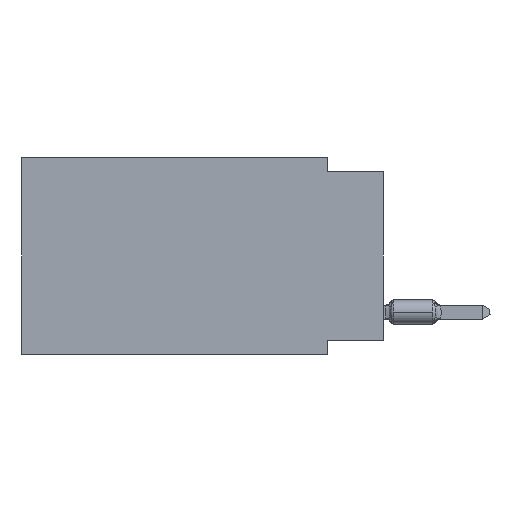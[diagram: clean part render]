
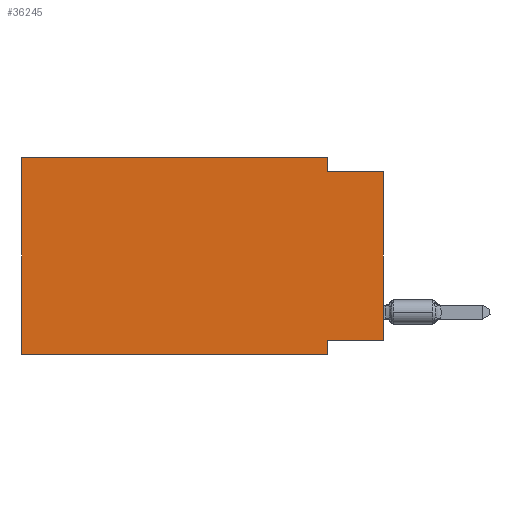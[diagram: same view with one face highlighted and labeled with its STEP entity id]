
A CAD part, left-side view. The second image highlights one B-rep face of the part: STEP entity #36245.
In plain terms, the highlighted planar face has unit normal (-1, 0, 0).
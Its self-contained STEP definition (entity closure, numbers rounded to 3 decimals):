
#801 = EDGE_CURVE ( 'NONE', #10428, #63160, #31707, .T. ) ;
#3510 = VECTOR ( 'NONE', #16672, 1000. ) ;
#4188 = CARTESIAN_POINT ( 'NONE',  ( 0., 0., -8.255 ) ) ;
#4580 = CARTESIAN_POINT ( 'NONE',  ( 0., 16.383, 0. ) ) ;
#5194 = FACE_OUTER_BOUND ( 'NONE', #32327, .T. ) ;
#7458 = CARTESIAN_POINT ( 'NONE',  ( 0., 0., -8.255 ) ) ;
#8635 = CARTESIAN_POINT ( 'NONE',  ( 0., 0., -0.635 ) ) ;
#9590 = CARTESIAN_POINT ( 'NONE',  ( 0., 16.383, 0. ) ) ;
#10428 = VERTEX_POINT ( 'NONE', #29338 ) ;
#11068 = CARTESIAN_POINT ( 'NONE',  ( 0., 2.54, -0.635 ) ) ;
#11115 = AXIS2_PLACEMENT_3D ( 'NONE', #39420, #14782, #29189 ) ;
#11839 = VERTEX_POINT ( 'NONE', #8635 ) ;
#14782 = DIRECTION ( 'NONE',  ( 1., 0., 0. ) ) ;
#16672 = DIRECTION ( 'NONE',  ( 0., 0., 1. ) ) ;
#18533 = LINE ( 'NONE', #28449, #47121 ) ;
#18869 = LINE ( 'NONE', #9590, #39000 ) ;
#18970 = ORIENTED_EDGE ( 'NONE', *, *, #21011, .F. ) ;
#19207 = CARTESIAN_POINT ( 'NONE',  ( 0., 2.54, 0. ) ) ;
#19904 = PLANE ( 'NONE',  #11115 ) ;
#20805 = DIRECTION ( 'NONE',  ( 0., 0., -1. ) ) ;
#21011 = EDGE_CURVE ( 'NONE', #24357, #11839, #50283, .T. ) ;
#21856 = EDGE_CURVE ( 'NONE', #10428, #28806, #18533, .T. ) ;
#22291 = VECTOR ( 'NONE', #33310, 1000. ) ;
#23144 = CARTESIAN_POINT ( 'NONE',  ( 0., 2.54, -8.89 ) ) ;
#23416 = ORIENTED_EDGE ( 'NONE', *, *, #34055, .F. ) ;
#24179 = CARTESIAN_POINT ( 'NONE',  ( 0., 2.54, -8.255 ) ) ;
#24357 = VERTEX_POINT ( 'NONE', #11068 ) ;
#26567 = DIRECTION ( 'NONE',  ( 0., -1., 0. ) ) ;
#28449 = CARTESIAN_POINT ( 'NONE',  ( 0., 16.383, -8.89 ) ) ;
#28806 = VERTEX_POINT ( 'NONE', #23144 ) ;
#29101 = DIRECTION ( 'NONE',  ( 0., -1., 0. ) ) ;
#29189 = DIRECTION ( 'NONE',  ( 0., 0., -1. ) ) ;
#29338 = CARTESIAN_POINT ( 'NONE',  ( 0., 16.383, -8.89 ) ) ;
#31707 = LINE ( 'NONE', #50925, #3510 ) ;
#32327 = EDGE_LOOP ( 'NONE', ( #61932, #18970, #61066, #52282, #50179, #55078, #33353, #23416 ) ) ;
#33310 = DIRECTION ( 'NONE',  ( 0., 1., 0. ) ) ;
#33353 = ORIENTED_EDGE ( 'NONE', *, *, #44861, .F. ) ;
#33989 = LINE ( 'NONE', #49350, #41806 ) ;
#34055 = EDGE_CURVE ( 'NONE', #34829, #39649, #52845, .T. ) ;
#34829 = VERTEX_POINT ( 'NONE', #7458 ) ;
#34842 = CARTESIAN_POINT ( 'NONE',  ( 0., 2.54, -8.89 ) ) ;
#34889 = CARTESIAN_POINT ( 'NONE',  ( 0., 2.54, 0. ) ) ;
#36245 = ADVANCED_FACE ( 'NONE', ( #5194 ), #19904, .F. ) ;
#36271 = EDGE_CURVE ( 'NONE', #34829, #11839, #33989, .T. ) ;
#36630 = VERTEX_POINT ( 'NONE', #19207 ) ;
#37724 = VECTOR ( 'NONE', #26567, 1000. ) ;
#39000 = VECTOR ( 'NONE', #29101, 1000. ) ;
#39420 = CARTESIAN_POINT ( 'NONE',  ( 0., 16.383, 0. ) ) ;
#39649 = VERTEX_POINT ( 'NONE', #24179 ) ;
#40978 = LINE ( 'NONE', #34889, #50881 ) ;
#41806 = VECTOR ( 'NONE', #49029, 1000. ) ;
#44258 = EDGE_CURVE ( 'NONE', #63160, #36630, #18869, .T. ) ;
#44861 = EDGE_CURVE ( 'NONE', #39649, #28806, #59173, .T. ) ;
#45470 = CARTESIAN_POINT ( 'NONE',  ( 0., 0., -0.635 ) ) ;
#47121 = VECTOR ( 'NONE', #48605, 1000. ) ;
#48605 = DIRECTION ( 'NONE',  ( 0., -1., 0. ) ) ;
#49029 = DIRECTION ( 'NONE',  ( 0., 0., 1. ) ) ;
#49350 = CARTESIAN_POINT ( 'NONE',  ( 0., 0., 0. ) ) ;
#50179 = ORIENTED_EDGE ( 'NONE', *, *, #801, .F. ) ;
#50283 = LINE ( 'NONE', #45470, #37724 ) ;
#50335 = VECTOR ( 'NONE', #54371, 1000. ) ;
#50881 = VECTOR ( 'NONE', #20805, 1000. ) ;
#50925 = CARTESIAN_POINT ( 'NONE',  ( 0., 16.383, 0. ) ) ;
#52282 = ORIENTED_EDGE ( 'NONE', *, *, #44258, .F. ) ;
#52845 = LINE ( 'NONE', #4188, #22291 ) ;
#54371 = DIRECTION ( 'NONE',  ( 0., 0., -1. ) ) ;
#55078 = ORIENTED_EDGE ( 'NONE', *, *, #21856, .T. ) ;
#58004 = EDGE_CURVE ( 'NONE', #36630, #24357, #40978, .T. ) ;
#59173 = LINE ( 'NONE', #34842, #50335 ) ;
#61066 = ORIENTED_EDGE ( 'NONE', *, *, #58004, .F. ) ;
#61932 = ORIENTED_EDGE ( 'NONE', *, *, #36271, .T. ) ;
#63160 = VERTEX_POINT ( 'NONE', #4580 ) ;
